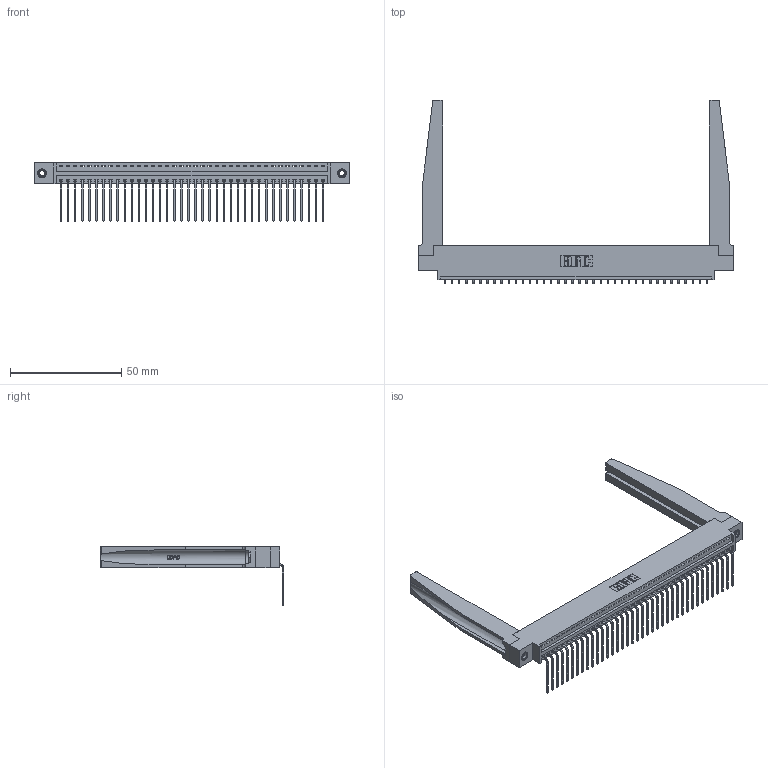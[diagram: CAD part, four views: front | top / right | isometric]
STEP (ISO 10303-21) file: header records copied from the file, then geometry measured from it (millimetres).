
FILE_DESCRIPTION (( 'STEP AP203' ), '1' );
FILE_NAME ('346-038-559-678.STEP', '2022-05-07T06:02:19', ( '' ), ( '' ), 'SwSTEP 2.0', 'SolidWorks 2020', '' );
FILE_SCHEMA (( 'CONFIG_CONTROL_DESIGN' ));
Length unit declared in the file: inch
Products named in the file (5): 346 Part_0.170 Offset - 0.156 Dia-TH; 346-038-559-678; 346-220-078_345-220-078; 345-250-001_345-250-001-102; 345-292-001_558 559 Tail - 1
Assembly tree (43 placements, depth 2):
  346-038-559-678
    346 Part_0.170 Offset - 0.156 Dia-TH
    345-292-001_558 559 Tail - 1  x38
    346-220-078_345-220-078  x2
    345-250-001_345-250-001-102  x2
Bounding box: 141.22 x 82.36 x 26.16 mm (x, y, z)
Volume: 20353.5 mm3; surface area: 24248.9 mm2
Topology: 43 solids, 43 shells, 2654 faces, 7901 edges, 5206 vertices
Faces by surface type: plane 1832, cylinder 770, bspline 36, cone 12, torus 4
Entity records: 29502 total; most frequent: CARTESIAN_POINT 5975, ORIENTED_EDGE 4834, DIRECTION 4259, EDGE_CURVE 2417, LINE 2039, VECTOR 2039, VERTEX_POINT 1604, AXIS2_PLACEMENT_3D 1110
